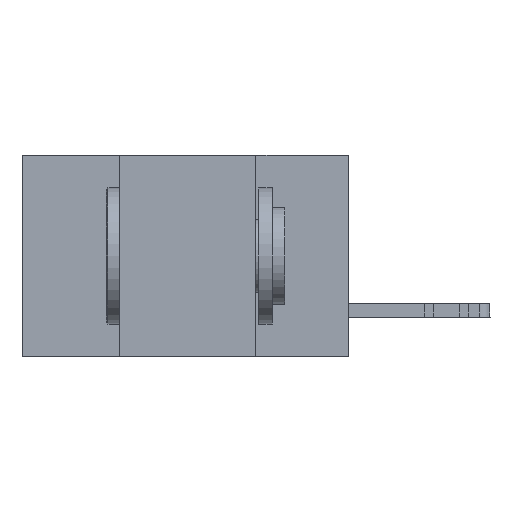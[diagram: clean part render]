
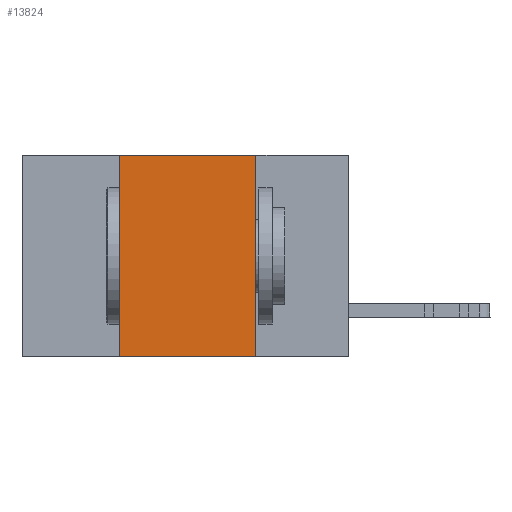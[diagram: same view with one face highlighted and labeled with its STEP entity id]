
A CAD part, left-side view. The second image highlights one B-rep face of the part: STEP entity #13824.
In plain terms, the highlighted planar face has unit normal (-1, 0, 0).
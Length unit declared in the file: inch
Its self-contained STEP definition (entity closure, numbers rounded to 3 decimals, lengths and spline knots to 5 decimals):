
#347 = VECTOR ( 'NONE', #21959, 39.37008 ) ;
#574 = PLANE ( 'NONE',  #13755 ) ;
#1079 = VERTEX_POINT ( 'NONE', #11607 ) ;
#2777 = CARTESIAN_POINT ( 'NONE',  ( 0., 0.6, 0. ) ) ;
#3916 = VERTEX_POINT ( 'NONE', #21234 ) ;
#5872 = LINE ( 'NONE', #18450, #26093 ) ;
#6934 = LINE ( 'NONE', #28403, #347 ) ;
#7109 = VECTOR ( 'NONE', #25334, 39.37008 ) ;
#7777 = FACE_OUTER_BOUND ( 'NONE', #16501, .T. ) ;
#7932 = ORIENTED_EDGE ( 'NONE', *, *, #16263, .F. ) ;
#9129 = VERTEX_POINT ( 'NONE', #13834 ) ;
#9952 = VERTEX_POINT ( 'NONE', #11972 ) ;
#11607 = CARTESIAN_POINT ( 'NONE',  ( 0., 0.17, 0. ) ) ;
#11680 = DIRECTION ( 'NONE',  ( 0., 0., 1. ) ) ;
#11794 = ORIENTED_EDGE ( 'NONE', *, *, #16921, .F. ) ;
#11877 = CARTESIAN_POINT ( 'NONE',  ( 0., 0.17, 0. ) ) ;
#11972 = CARTESIAN_POINT ( 'NONE',  ( 0., 0.17, -0.37 ) ) ;
#13054 = LINE ( 'NONE', #11877, #7109 ) ;
#13214 = DIRECTION ( 'NONE',  ( 0., 0., -1. ) ) ;
#13755 = AXIS2_PLACEMENT_3D ( 'NONE', #2777, #18401, #13214 ) ;
#13824 = ADVANCED_FACE ( 'NONE', ( #7777 ), #574, .F. ) ;
#13834 = CARTESIAN_POINT ( 'NONE',  ( 0., 0.42, -0.37 ) ) ;
#16263 = EDGE_CURVE ( 'NONE', #3916, #1079, #6934, .T. ) ;
#16501 = EDGE_LOOP ( 'NONE', ( #21558, #7932, #11794, #25958 ) ) ;
#16921 = EDGE_CURVE ( 'NONE', #9129, #3916, #5872, .T. ) ;
#16956 = DIRECTION ( 'NONE',  ( 0., -1., 0. ) ) ;
#18401 = DIRECTION ( 'NONE',  ( 1., 0., 0. ) ) ;
#18450 = CARTESIAN_POINT ( 'NONE',  ( 0., 0.42, 0. ) ) ;
#19578 = EDGE_CURVE ( 'NONE', #1079, #9952, #13054, .T. ) ;
#21234 = CARTESIAN_POINT ( 'NONE',  ( 0., 0.42, 0. ) ) ;
#21558 = ORIENTED_EDGE ( 'NONE', *, *, #19578, .F. ) ;
#21959 = DIRECTION ( 'NONE',  ( 0., -1., 0. ) ) ;
#22222 = VECTOR ( 'NONE', #16956, 39.37008 ) ;
#25334 = DIRECTION ( 'NONE',  ( 0., 0., -1. ) ) ;
#25958 = ORIENTED_EDGE ( 'NONE', *, *, #27388, .T. ) ;
#26093 = VECTOR ( 'NONE', #11680, 39.37008 ) ;
#27388 = EDGE_CURVE ( 'NONE', #9129, #9952, #28155, .T. ) ;
#27538 = CARTESIAN_POINT ( 'NONE',  ( 0., 0.6, -0.37 ) ) ;
#28155 = LINE ( 'NONE', #27538, #22222 ) ;
#28403 = CARTESIAN_POINT ( 'NONE',  ( 0., 0.6, 0. ) ) ;
